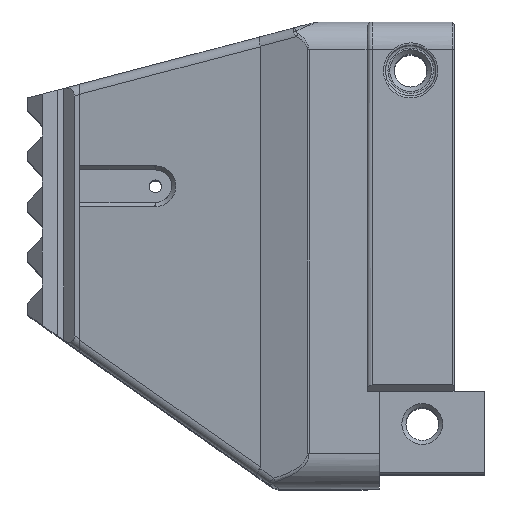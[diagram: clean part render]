
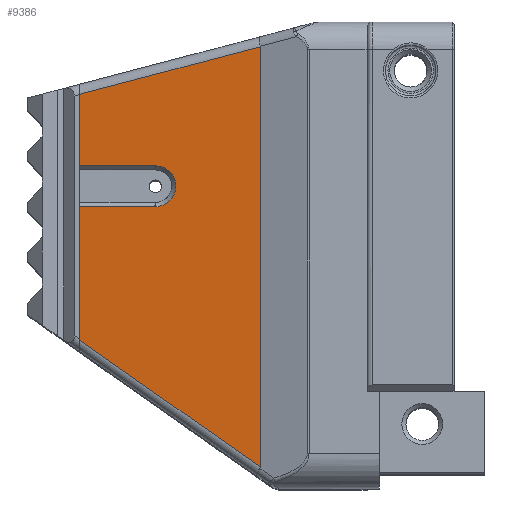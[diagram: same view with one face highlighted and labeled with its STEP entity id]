
A CAD part, top view. The second image highlights one B-rep face of the part: STEP entity #9386.
In plain terms, the highlighted planar face has unit normal (-0.138, 0, 0.99).
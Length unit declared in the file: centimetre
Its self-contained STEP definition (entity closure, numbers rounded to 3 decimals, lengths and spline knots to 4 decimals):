
#811=B_SPLINE_CURVE_WITH_KNOTS($,3,(#16959,#16960,#16961,#16962,#16963,
#16964,#16965,#16966),.UNSPECIFIED.,.F.,.F.,(4,1,1,1,1,4),(-1.5708,
-0.6732,0.2244,0.6732,1.122,
1.5708),.UNSPECIFIED.);
#813=B_SPLINE_CURVE_WITH_KNOTS($,3,(#16993,#16994,#16995,#16996),
 .UNSPECIFIED.,.F.,.F.,(4,4),(-1.2115,-1.2003),
 .UNSPECIFIED.);
#815=B_SPLINE_CURVE_WITH_KNOTS($,3,(#17026,#17027,#17028,#17029),
 .UNSPECIFIED.,.F.,.F.,(4,4),(1.2003,1.2115),
 .UNSPECIFIED.);
#1290=FACE_OUTER_BOUND($,#1922,.T.);
#1922=EDGE_LOOP($,(#7684,#7685,#7686,#7687,#7688,#7689,#7690,#7691,#7692,
#7693));
#2698=LINE($,#16922,#3523);
#2702=LINE($,#17006,#3527);
#2705=LINE($,#17036,#3530);
#2706=LINE($,#17038,#3531);
#2707=LINE($,#17040,#3532);
#2708=LINE($,#17042,#3533);
#2709=LINE($,#17043,#3534);
#3523=VECTOR($,#12087,1.5034);
#3527=VECTOR($,#12093,1.5034);
#3530=VECTOR($,#12098,2.6491);
#3531=VECTOR($,#12099,4.4048);
#3532=VECTOR($,#12100,8.3386);
#3533=VECTOR($,#12101,3.7355);
#3534=VECTOR($,#12102,1.4202);
#4381=VERTEX_POINT($,#16915);
#4384=VERTEX_POINT($,#16920);
#4386=VERTEX_POINT($,#16956);
#4387=VERTEX_POINT($,#16958);
#4390=VERTEX_POINT($,#17003);
#4391=VERTEX_POINT($,#17005);
#4393=VERTEX_POINT($,#17035);
#4394=VERTEX_POINT($,#17037);
#4395=VERTEX_POINT($,#17039);
#4396=VERTEX_POINT($,#17041);
#5536=EDGE_CURVE($,#4384,#4381,#2698,.T.);
#5538=EDGE_CURVE($,#4386,#4387,#811,.T.);
#5541=EDGE_CURVE($,#4387,#4384,#813,.T.);
#5544=EDGE_CURVE($,#4390,#4391,#2702,.T.);
#5547=EDGE_CURVE($,#4391,#4386,#815,.T.);
#5549=EDGE_CURVE($,#4393,#4390,#2705,.T.);
#5550=EDGE_CURVE($,#4394,#4393,#2706,.T.);
#5551=EDGE_CURVE($,#4394,#4395,#2707,.F.);
#5552=EDGE_CURVE($,#4396,#4395,#2708,.T.);
#5553=EDGE_CURVE($,#4381,#4396,#2709,.T.);
#7684=ORIENTED_EDGE($,*,*,#5536,.F.);
#7685=ORIENTED_EDGE($,*,*,#5541,.F.);
#7686=ORIENTED_EDGE($,*,*,#5538,.F.);
#7687=ORIENTED_EDGE($,*,*,#5547,.F.);
#7688=ORIENTED_EDGE($,*,*,#5544,.F.);
#7689=ORIENTED_EDGE($,*,*,#5549,.F.);
#7690=ORIENTED_EDGE($,*,*,#5550,.F.);
#7691=ORIENTED_EDGE($,*,*,#5551,.T.);
#7692=ORIENTED_EDGE($,*,*,#5552,.F.);
#7693=ORIENTED_EDGE($,*,*,#5553,.F.);
#8928=PLANE($,#10154);
#9386=ADVANCED_FACE($,(#1290),#8928,.F.);
#10154=AXIS2_PLACEMENT_3D($,#17034,#12096,#12097);
#12087=DIRECTION($,(-0.99,0.,-0.138));
#12093=DIRECTION($,(0.99,0.,0.138));
#12096=DIRECTION('center_axis',(0.138,0.,
-0.99));
#12097=DIRECTION('ref_axis',(-0.99,0.,
-0.138));
#12098=DIRECTION($,(0.,1.,0.));
#12099=DIRECTION($,(-0.813,0.571,-0.114));
#12100=DIRECTION($,(0.,-1.,0.));
#12101=DIRECTION($,(0.958,0.252,0.134));
#12102=DIRECTION($,(0.,1.,0.));
#16915=CARTESIAN_POINT('',(-25.2982,5.0571,11.1));
#16920=CARTESIAN_POINT('',(-23.8093,5.0571,11.3079));
#16922=CARTESIAN_POINT($,(-24.9981,5.0571,11.1419));
#16956=CARTESIAN_POINT('',(-23.7982,4.2471,11.3095));
#16958=CARTESIAN_POINT('',(-23.7982,5.0571,11.3095));
#16959=CARTESIAN_POINT('Ctrl Pts',(-23.7982,4.2471,11.3095));
#16960=CARTESIAN_POINT('Ctrl Pts',(-23.6775,4.2471,11.3264));
#16961=CARTESIAN_POINT('Ctrl Pts',(-23.4367,4.3635,11.36));
#16962=CARTESIAN_POINT('Ctrl Pts',(-23.3622,4.6897,11.3704));
#16963=CARTESIAN_POINT('Ctrl Pts',(-23.4719,4.9138,11.3551));
#16964=CARTESIAN_POINT('Ctrl Pts',(-23.6169,5.0296,11.3348));
#16965=CARTESIAN_POINT('Ctrl Pts',(-23.7378,5.0571,11.3179));
#16966=CARTESIAN_POINT('Ctrl Pts',(-23.7982,5.0571,11.3095));
#16993=CARTESIAN_POINT('Ctrl Pts',(-23.7982,5.0571,11.3095));
#16994=CARTESIAN_POINT('Ctrl Pts',(-23.8019,5.0571,11.309));
#16995=CARTESIAN_POINT('Ctrl Pts',(-23.8056,5.0571,11.3085));
#16996=CARTESIAN_POINT('Ctrl Pts',(-23.8093,5.0571,11.3079));
#17003=CARTESIAN_POINT('',(-25.2982,4.2471,11.1));
#17005=CARTESIAN_POINT('',(-23.8093,4.2471,11.3079));
#17006=CARTESIAN_POINT($,(-24.9981,4.2471,11.1419));
#17026=CARTESIAN_POINT('Ctrl Pts',(-23.8093,4.2471,11.3079));
#17027=CARTESIAN_POINT('Ctrl Pts',(-23.8056,4.2471,11.3085));
#17028=CARTESIAN_POINT('Ctrl Pts',(-23.8019,4.2471,11.309));
#17029=CARTESIAN_POINT('Ctrl Pts',(-23.7982,4.2471,11.3095));
#17034=CARTESIAN_POINT('Origin',(-26.2886,-1.3536,10.9617));
#17035=CARTESIAN_POINT('',(-25.2982,1.598,11.1));
#17036=CARTESIAN_POINT($,(-25.2982,1.7147,11.1));
#17037=CARTESIAN_POINT('',(-21.7182,-0.9191,11.6));
#17038=CARTESIAN_POINT($,(-26.5173,2.4552,10.9297));
#17039=CARTESIAN_POINT('',(-21.7182,7.4194,11.6));
#17040=CARTESIAN_POINT($,(-21.7182,-1.3536,11.6));
#17041=CARTESIAN_POINT('',(-25.2982,6.4773,11.1));
#17042=CARTESIAN_POINT($,(-27.2555,5.9623,10.8266));
#17043=CARTESIAN_POINT($,(-25.2982,1.7147,11.1));
